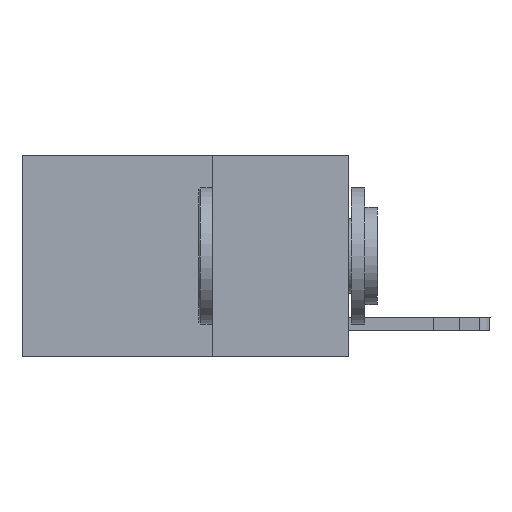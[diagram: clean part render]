
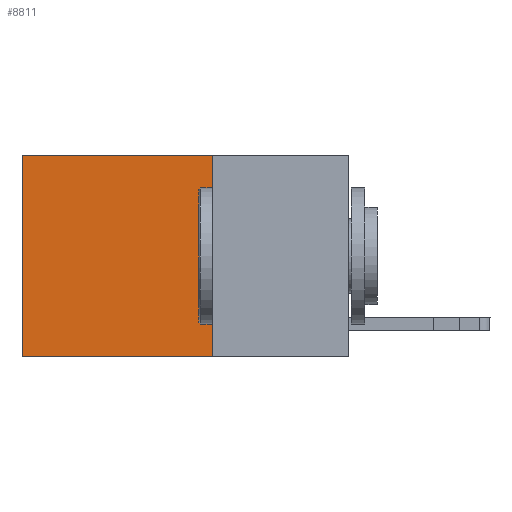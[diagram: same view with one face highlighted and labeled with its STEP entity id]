
A CAD part, left-side view. The second image highlights one B-rep face of the part: STEP entity #8811.
In plain terms, the highlighted planar face has unit normal (-1, 0, 0).
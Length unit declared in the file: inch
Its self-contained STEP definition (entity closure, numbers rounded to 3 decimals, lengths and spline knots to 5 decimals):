
#642 = DIRECTION ( 'NONE',  ( 0., 1., 0. ) ) ;
#782 = VECTOR ( 'NONE', #11714, 39.37008 ) ;
#2391 = VERTEX_POINT ( 'NONE', #8674 ) ;
#3019 = VECTOR ( 'NONE', #642, 39.37008 ) ;
#3060 = ORIENTED_EDGE ( 'NONE', *, *, #4384, .T. ) ;
#4262 = VERTEX_POINT ( 'NONE', #8846 ) ;
#4384 = EDGE_CURVE ( 'NONE', #16922, #2391, #13516, .T. ) ;
#4578 = EDGE_CURVE ( 'NONE', #4262, #2391, #14388, .T. ) ;
#5314 = AXIS2_PLACEMENT_3D ( 'NONE', #8839, #19302, #16371 ) ;
#6496 = DIRECTION ( 'NONE',  ( 0., 1., 0. ) ) ;
#6977 = CARTESIAN_POINT ( 'NONE',  ( 0.2625, 0.25, -0.37 ) ) ;
#7582 = DIRECTION ( 'NONE',  ( 0., 0., -1. ) ) ;
#7651 = VERTEX_POINT ( 'NONE', #10839 ) ;
#7956 = CARTESIAN_POINT ( 'NONE',  ( 0.2625, 0.6, 0. ) ) ;
#8674 = CARTESIAN_POINT ( 'NONE',  ( 0.2625, 0.6, -0.37 ) ) ;
#8741 = FACE_OUTER_BOUND ( 'NONE', #12736, .T. ) ;
#8811 = ADVANCED_FACE ( 'NONE', ( #8741 ), #10117, .F. ) ;
#8839 = CARTESIAN_POINT ( 'NONE',  ( 0.2625, 0.25, 0. ) ) ;
#8846 = CARTESIAN_POINT ( 'NONE',  ( 0.2625, 0.25, -0.37 ) ) ;
#9101 = VECTOR ( 'NONE', #6496, 39.37008 ) ;
#9154 = ORIENTED_EDGE ( 'NONE', *, *, #4578, .F. ) ;
#9230 = VECTOR ( 'NONE', #7582, 39.37008 ) ;
#10117 = PLANE ( 'NONE',  #5314 ) ;
#10621 = ORIENTED_EDGE ( 'NONE', *, *, #15482, .F. ) ;
#10785 = ORIENTED_EDGE ( 'NONE', *, *, #12488, .T. ) ;
#10839 = CARTESIAN_POINT ( 'NONE',  ( 0.2625, 0.25, 0. ) ) ;
#11714 = DIRECTION ( 'NONE',  ( 0., 0., -1. ) ) ;
#12488 = EDGE_CURVE ( 'NONE', #7651, #16922, #13804, .T. ) ;
#12736 = EDGE_LOOP ( 'NONE', ( #3060, #9154, #10621, #10785 ) ) ;
#13176 = CARTESIAN_POINT ( 'NONE',  ( 0.2625, 0.25, 0. ) ) ;
#13516 = LINE ( 'NONE', #7956, #9230 ) ;
#13804 = LINE ( 'NONE', #18535, #9101 ) ;
#14388 = LINE ( 'NONE', #6977, #3019 ) ;
#15482 = EDGE_CURVE ( 'NONE', #7651, #4262, #17628, .T. ) ;
#16371 = DIRECTION ( 'NONE',  ( 0., 0., -1. ) ) ;
#16922 = VERTEX_POINT ( 'NONE', #18216 ) ;
#17628 = LINE ( 'NONE', #13176, #782 ) ;
#18216 = CARTESIAN_POINT ( 'NONE',  ( 0.2625, 0.6, 0. ) ) ;
#18535 = CARTESIAN_POINT ( 'NONE',  ( 0.2625, 0.25, 0. ) ) ;
#19302 = DIRECTION ( 'NONE',  ( 1., 0., 0. ) ) ;
